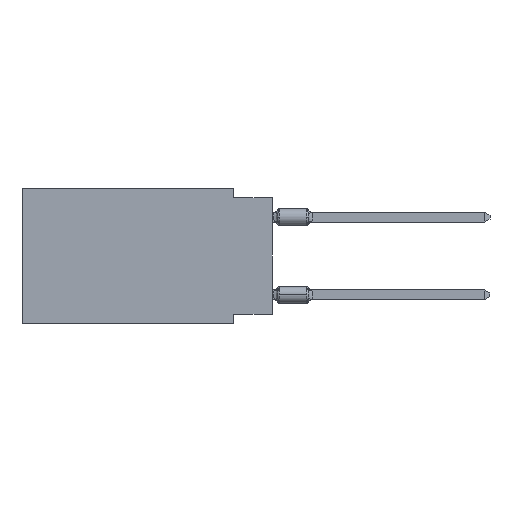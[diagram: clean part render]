
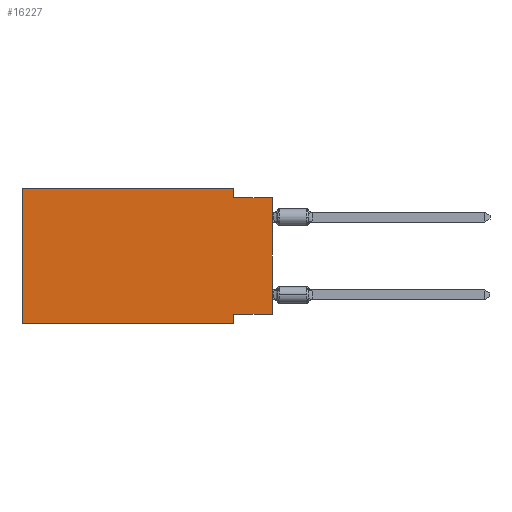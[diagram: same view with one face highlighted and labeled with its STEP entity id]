
A CAD part, left-side view. The second image highlights one B-rep face of the part: STEP entity #16227.
In plain terms, the highlighted planar face has unit normal (-1, 0, 0).
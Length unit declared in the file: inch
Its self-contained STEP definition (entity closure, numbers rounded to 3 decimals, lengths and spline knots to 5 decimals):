
#302 = CARTESIAN_POINT ( 'NONE',  ( 0., 0.645, 0. ) ) ;
#1100 = DIRECTION ( 'NONE',  ( 0., 0., 1. ) ) ;
#1544 = EDGE_CURVE ( 'NONE', #9434, #6620, #7509, .T. ) ;
#1732 = DIRECTION ( 'NONE',  ( 0., -1., 0. ) ) ;
#2509 = CARTESIAN_POINT ( 'NONE',  ( 0., 0.645, 0. ) ) ;
#2601 = LINE ( 'NONE', #19069, #7768 ) ;
#2675 = VERTEX_POINT ( 'NONE', #12450 ) ;
#3133 = EDGE_CURVE ( 'NONE', #14228, #19348, #8924, .T. ) ;
#3651 = PLANE ( 'NONE',  #9344 ) ;
#3917 = CARTESIAN_POINT ( 'NONE',  ( 0., 0.645, 0. ) ) ;
#4497 = ORIENTED_EDGE ( 'NONE', *, *, #1544, .F. ) ;
#4587 = VECTOR ( 'NONE', #1100, 39.37008 ) ;
#4621 = VECTOR ( 'NONE', #8902, 39.37008 ) ;
#4720 = ORIENTED_EDGE ( 'NONE', *, *, #9197, .F. ) ;
#4947 = CARTESIAN_POINT ( 'NONE',  ( 0., 0., -0.025 ) ) ;
#5083 = VECTOR ( 'NONE', #20194, 39.37008 ) ;
#5238 = CARTESIAN_POINT ( 'NONE',  ( 0., 0., -0.025 ) ) ;
#5452 = VECTOR ( 'NONE', #7477, 39.37008 ) ;
#5527 = CARTESIAN_POINT ( 'NONE',  ( 0., 0.1, 0. ) ) ;
#5833 = CARTESIAN_POINT ( 'NONE',  ( 0., 0.1, -0.35 ) ) ;
#6063 = DIRECTION ( 'NONE',  ( 0., -1., 0. ) ) ;
#6279 = CARTESIAN_POINT ( 'NONE',  ( 0., 0.645, 0. ) ) ;
#6620 = VERTEX_POINT ( 'NONE', #3917 ) ;
#6775 = EDGE_CURVE ( 'NONE', #6620, #14228, #19587, .T. ) ;
#7387 = DIRECTION ( 'NONE',  ( 0., 0., 1. ) ) ;
#7477 = DIRECTION ( 'NONE',  ( 0., 0., -1. ) ) ;
#7509 = LINE ( 'NONE', #2509, #4587 ) ;
#7768 = VECTOR ( 'NONE', #7387, 39.37008 ) ;
#7938 = VECTOR ( 'NONE', #20361, 39.37008 ) ;
#8690 = CARTESIAN_POINT ( 'NONE',  ( 0., 0., -0.325 ) ) ;
#8902 = DIRECTION ( 'NONE',  ( 0., 1., 0. ) ) ;
#8924 = LINE ( 'NONE', #5527, #7938 ) ;
#9080 = EDGE_CURVE ( 'NONE', #19348, #13598, #11919, .T. ) ;
#9197 = EDGE_CURVE ( 'NONE', #21221, #2675, #9223, .T. ) ;
#9223 = LINE ( 'NONE', #5833, #5452 ) ;
#9344 = AXIS2_PLACEMENT_3D ( 'NONE', #302, #18272, #10421 ) ;
#9434 = VERTEX_POINT ( 'NONE', #14227 ) ;
#9951 = ORIENTED_EDGE ( 'NONE', *, *, #17412, .F. ) ;
#10421 = DIRECTION ( 'NONE',  ( 0., 0., -1. ) ) ;
#11919 = LINE ( 'NONE', #5238, #5083 ) ;
#12450 = CARTESIAN_POINT ( 'NONE',  ( 0., 0.1, -0.35 ) ) ;
#12732 = CARTESIAN_POINT ( 'NONE',  ( 0., 0., -0.325 ) ) ;
#12735 = VECTOR ( 'NONE', #6063, 39.37008 ) ;
#12946 = CARTESIAN_POINT ( 'NONE',  ( 0., 0.645, -0.35 ) ) ;
#13284 = CARTESIAN_POINT ( 'NONE',  ( 0., 0.1, -0.325 ) ) ;
#13503 = VERTEX_POINT ( 'NONE', #12732 ) ;
#13598 = VERTEX_POINT ( 'NONE', #4947 ) ;
#14074 = VECTOR ( 'NONE', #1732, 39.37008 ) ;
#14174 = ORIENTED_EDGE ( 'NONE', *, *, #9080, .F. ) ;
#14227 = CARTESIAN_POINT ( 'NONE',  ( 0., 0.645, -0.35 ) ) ;
#14228 = VERTEX_POINT ( 'NONE', #17692 ) ;
#14979 = ORIENTED_EDGE ( 'NONE', *, *, #17375, .T. ) ;
#16227 = ADVANCED_FACE ( 'NONE', ( #20444 ), #3651, .F. ) ;
#16612 = ORIENTED_EDGE ( 'NONE', *, *, #17234, .T. ) ;
#17234 = EDGE_CURVE ( 'NONE', #13503, #13598, #2601, .T. ) ;
#17375 = EDGE_CURVE ( 'NONE', #9434, #2675, #18073, .T. ) ;
#17412 = EDGE_CURVE ( 'NONE', #13503, #21221, #18506, .T. ) ;
#17692 = CARTESIAN_POINT ( 'NONE',  ( 0., 0.1, 0. ) ) ;
#18073 = LINE ( 'NONE', #12946, #14074 ) ;
#18123 = CARTESIAN_POINT ( 'NONE',  ( 0., 0.1, -0.025 ) ) ;
#18124 = EDGE_LOOP ( 'NONE', ( #16612, #14174, #19294, #20937, #4497, #14979, #4720, #9951 ) ) ;
#18272 = DIRECTION ( 'NONE',  ( 1., 0., 0. ) ) ;
#18506 = LINE ( 'NONE', #8690, #4621 ) ;
#19069 = CARTESIAN_POINT ( 'NONE',  ( 0., 0., 0. ) ) ;
#19294 = ORIENTED_EDGE ( 'NONE', *, *, #3133, .F. ) ;
#19348 = VERTEX_POINT ( 'NONE', #18123 ) ;
#19587 = LINE ( 'NONE', #6279, #12735 ) ;
#20194 = DIRECTION ( 'NONE',  ( 0., -1., 0. ) ) ;
#20361 = DIRECTION ( 'NONE',  ( 0., 0., -1. ) ) ;
#20444 = FACE_OUTER_BOUND ( 'NONE', #18124, .T. ) ;
#20937 = ORIENTED_EDGE ( 'NONE', *, *, #6775, .F. ) ;
#21221 = VERTEX_POINT ( 'NONE', #13284 ) ;
